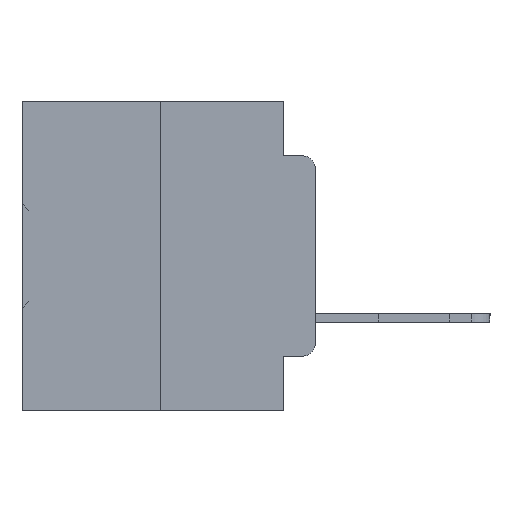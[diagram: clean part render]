
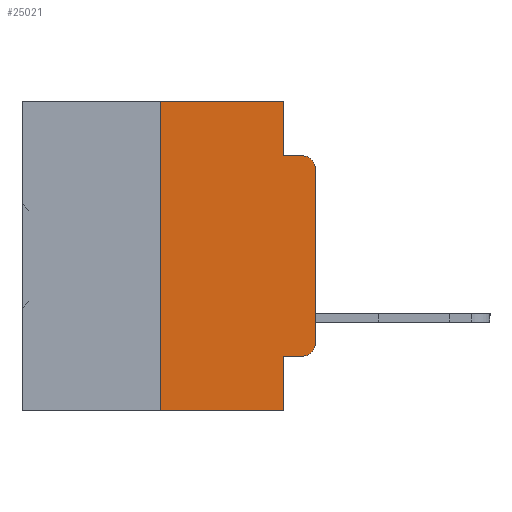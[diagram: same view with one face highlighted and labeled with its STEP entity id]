
A CAD part, left-side view. The second image highlights one B-rep face of the part: STEP entity #25021.
In plain terms, the highlighted planar face has unit normal (-1, 0, 0).
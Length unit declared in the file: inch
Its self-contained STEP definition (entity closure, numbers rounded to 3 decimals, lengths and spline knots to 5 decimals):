
#84 = DIRECTION ( 'NONE',  ( -1., 0., 0. ) ) ;
#321 = VERTEX_POINT ( 'NONE', #16302 ) ;
#587 = ORIENTED_EDGE ( 'NONE', *, *, #3698, .F. ) ;
#841 = CARTESIAN_POINT ( 'NONE',  ( 0., 0.02, -0.3915 ) ) ;
#1013 = LINE ( 'NONE', #36197, #15486 ) ;
#1462 = CARTESIAN_POINT ( 'NONE',  ( 0., 0.02, -0.0885 ) ) ;
#1567 = EDGE_CURVE ( 'NONE', #25927, #19326, #17326, .T. ) ;
#1804 = CARTESIAN_POINT ( 'NONE',  ( 0., 0.25, -0.5 ) ) ;
#1955 = CARTESIAN_POINT ( 'NONE',  ( 0., 0.051, -0.4115 ) ) ;
#2072 = PLANE ( 'NONE',  #21960 ) ;
#3090 = CARTESIAN_POINT ( 'NONE',  ( 0., 0.473, -0.5 ) ) ;
#3669 = ORIENTED_EDGE ( 'NONE', *, *, #17635, .F. ) ;
#3698 = EDGE_CURVE ( 'NONE', #20939, #19662, #1013, .T. ) ;
#3749 = EDGE_CURVE ( 'NONE', #321, #27411, #16384, .T. ) ;
#4093 = VERTEX_POINT ( 'NONE', #20458 ) ;
#4277 = CARTESIAN_POINT ( 'NONE',  ( 0., 0.25, 0. ) ) ;
#5156 = VERTEX_POINT ( 'NONE', #4277 ) ;
#5193 = VERTEX_POINT ( 'NONE', #1804 ) ;
#7433 = LINE ( 'NONE', #27034, #37046 ) ;
#8516 = EDGE_CURVE ( 'NONE', #19326, #11190, #25919, .T. ) ;
#8682 = VECTOR ( 'NONE', #27694, 39.37008 ) ;
#8885 = DIRECTION ( 'NONE',  ( 0., -1., 0. ) ) ;
#9570 = LINE ( 'NONE', #17988, #31592 ) ;
#10879 = CARTESIAN_POINT ( 'NONE',  ( 0., 0.473, 0. ) ) ;
#11190 = VERTEX_POINT ( 'NONE', #1462 ) ;
#11384 = AXIS2_PLACEMENT_3D ( 'NONE', #17414, #84, #20265 ) ;
#12266 = DIRECTION ( 'NONE',  ( 0., 0., -1. ) ) ;
#12723 = DIRECTION ( 'NONE',  ( 0., -1., 0. ) ) ;
#13845 = DIRECTION ( 'NONE',  ( 0., 0., -1. ) ) ;
#14793 = CARTESIAN_POINT ( 'NONE',  ( 0., 0.051, -0.0885 ) ) ;
#15486 = VECTOR ( 'NONE', #12266, 39.37008 ) ;
#15804 = CIRCLE ( 'NONE', #11384, 0.02 ) ;
#16302 = CARTESIAN_POINT ( 'NONE',  ( 0., 0.02, -0.4115 ) ) ;
#16384 = CIRCLE ( 'NONE', #28281, 0.02 ) ;
#17319 = LINE ( 'NONE', #19190, #8682 ) ;
#17326 = LINE ( 'NONE', #35353, #28947 ) ;
#17414 = CARTESIAN_POINT ( 'NONE',  ( 0., 0.02, -0.1085 ) ) ;
#17635 = EDGE_CURVE ( 'NONE', #5156, #25927, #7433, .T. ) ;
#17713 = DIRECTION ( 'NONE',  ( 0., -1., 0. ) ) ;
#17988 = CARTESIAN_POINT ( 'NONE',  ( 0., 0., 0. ) ) ;
#18885 = CARTESIAN_POINT ( 'NONE',  ( 0., 0., -0.3915 ) ) ;
#19073 = EDGE_CURVE ( 'NONE', #5193, #5156, #17319, .T. ) ;
#19190 = CARTESIAN_POINT ( 'NONE',  ( 0., 0.25, 0. ) ) ;
#19326 = VERTEX_POINT ( 'NONE', #31649 ) ;
#19662 = VERTEX_POINT ( 'NONE', #33747 ) ;
#19946 = ORIENTED_EDGE ( 'NONE', *, *, #19073, .F. ) ;
#20140 = DIRECTION ( 'NONE',  ( -1., 0., 0. ) ) ;
#20265 = DIRECTION ( 'NONE',  ( 0., 0., -1. ) ) ;
#20416 = ORIENTED_EDGE ( 'NONE', *, *, #1567, .F. ) ;
#20458 = CARTESIAN_POINT ( 'NONE',  ( 0., 0., -0.1085 ) ) ;
#20835 = DIRECTION ( 'NONE',  ( 0., 0., 1. ) ) ;
#20939 = VERTEX_POINT ( 'NONE', #1955 ) ;
#21168 = ORIENTED_EDGE ( 'NONE', *, *, #29973, .T. ) ;
#21653 = FACE_OUTER_BOUND ( 'NONE', #24321, .T. ) ;
#21957 = CARTESIAN_POINT ( 'NONE',  ( 0., 0.051, -0.4115 ) ) ;
#21960 = AXIS2_PLACEMENT_3D ( 'NONE', #10879, #30999, #13845 ) ;
#23130 = ORIENTED_EDGE ( 'NONE', *, *, #35922, .T. ) ;
#24041 = ORIENTED_EDGE ( 'NONE', *, *, #35976, .T. ) ;
#24321 = EDGE_LOOP ( 'NONE', ( #21168, #23130, #36412, #20416, #3669, #19946, #24041, #587, #25297, #34204 ) ) ;
#24838 = DIRECTION ( 'NONE',  ( 0., -1., 0. ) ) ;
#25021 = ADVANCED_FACE ( 'NONE', ( #21653 ), #2072, .F. ) ;
#25023 = VECTOR ( 'NONE', #17713, 39.37008 ) ;
#25297 = ORIENTED_EDGE ( 'NONE', *, *, #28104, .T. ) ;
#25919 = LINE ( 'NONE', #14793, #25023 ) ;
#25927 = VERTEX_POINT ( 'NONE', #26689 ) ;
#26689 = CARTESIAN_POINT ( 'NONE',  ( 0., 0.051, 0. ) ) ;
#27034 = CARTESIAN_POINT ( 'NONE',  ( 0., 0.473, 0. ) ) ;
#27411 = VERTEX_POINT ( 'NONE', #18885 ) ;
#27694 = DIRECTION ( 'NONE',  ( 0., 0., 1. ) ) ;
#28104 = EDGE_CURVE ( 'NONE', #20939, #321, #35683, .T. ) ;
#28281 = AXIS2_PLACEMENT_3D ( 'NONE', #841, #20140, #34158 ) ;
#28947 = VECTOR ( 'NONE', #33924, 39.37008 ) ;
#29243 = LINE ( 'NONE', #3090, #35900 ) ;
#29973 = EDGE_CURVE ( 'NONE', #27411, #4093, #9570, .T. ) ;
#30999 = DIRECTION ( 'NONE',  ( 1., 0., 0. ) ) ;
#31592 = VECTOR ( 'NONE', #20835, 39.37008 ) ;
#31649 = CARTESIAN_POINT ( 'NONE',  ( 0., 0.051, -0.0885 ) ) ;
#33747 = CARTESIAN_POINT ( 'NONE',  ( 0., 0.051, -0.5 ) ) ;
#33924 = DIRECTION ( 'NONE',  ( 0., 0., -1. ) ) ;
#34158 = DIRECTION ( 'NONE',  ( 0., 0., -1. ) ) ;
#34204 = ORIENTED_EDGE ( 'NONE', *, *, #3749, .T. ) ;
#34802 = VECTOR ( 'NONE', #24838, 39.37008 ) ;
#35353 = CARTESIAN_POINT ( 'NONE',  ( 0., 0.051, 0. ) ) ;
#35683 = LINE ( 'NONE', #21957, #34802 ) ;
#35900 = VECTOR ( 'NONE', #8885, 39.37008 ) ;
#35922 = EDGE_CURVE ( 'NONE', #4093, #11190, #15804, .T. ) ;
#35976 = EDGE_CURVE ( 'NONE', #5193, #19662, #29243, .T. ) ;
#36197 = CARTESIAN_POINT ( 'NONE',  ( 0., 0.051, 0. ) ) ;
#36412 = ORIENTED_EDGE ( 'NONE', *, *, #8516, .F. ) ;
#37046 = VECTOR ( 'NONE', #12723, 39.37008 ) ;
